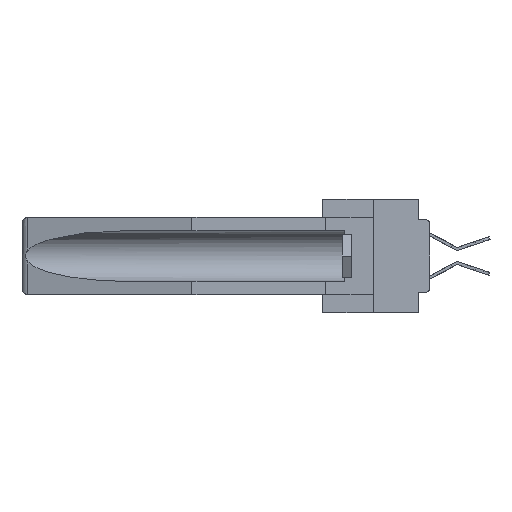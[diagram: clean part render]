
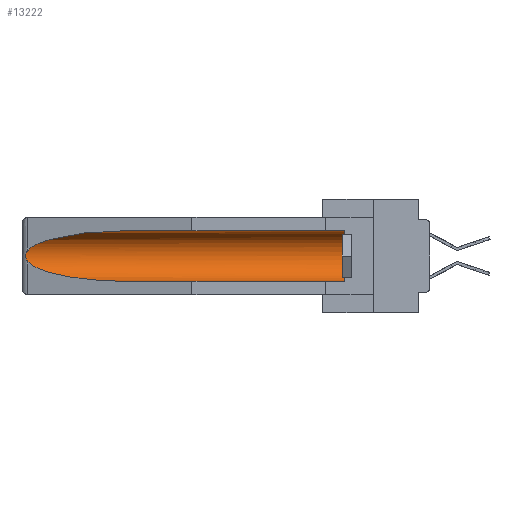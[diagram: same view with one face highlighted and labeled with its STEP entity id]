
A CAD part, left-side view. The second image highlights one B-rep face of the part: STEP entity #13222.
In plain terms, the highlighted cylindrical face has radius 2.857 mm (diameter 5.715 mm), a partial arc.
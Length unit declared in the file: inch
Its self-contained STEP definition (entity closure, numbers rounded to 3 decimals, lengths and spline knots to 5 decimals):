
#59 = CYLINDRICAL_SURFACE ( 'NONE', #3609, 0.1125 ) ;
#587 = CARTESIAN_POINT ( 'NONE',  ( 0.155, 0.126, -0.284 ) ) ;
#2237 = ORIENTED_EDGE ( 'NONE', *, *, #24105, .T. ) ;
#3097 = CARTESIAN_POINT ( 'NONE',  ( 0.26537, 1.52718, -0.19328 ) ) ;
#3282 = VECTOR ( 'NONE', #11240, 39.37008 ) ;
#3609 = AXIS2_PLACEMENT_3D ( 'NONE', #10146, #29214, #24515 ) ;
#4091 = CIRCLE ( 'NONE', #30299, 0.1125 ) ;
#4352 = CARTESIAN_POINT ( 'NONE',  ( 0.155, 1.07973, -0.059 ) ) ;
#4492 = VERTEX_POINT ( 'NONE', #15584 ) ;
#4972 = CARTESIAN_POINT ( 'NONE',  ( 0.26655, 1.53094, -0.18657 ) ) ;
#6360 = EDGE_LOOP ( 'NONE', ( #16870, #11389, #2237, #26771, #13676, #27246 ) ) ;
#6765 = CARTESIAN_POINT ( 'NONE',  ( 0.21114, 1.30732, -0.059 ) ) ;
#6907 = CARTESIAN_POINT ( 'NONE',  ( 0.26597, 1.52961, -0.15275 ) ) ;
#7057 = CARTESIAN_POINT ( 'NONE',  ( 0.2675, 1.53308, -0.17534 ) ) ;
#7318 = CARTESIAN_POINT ( 'NONE',  ( 0.26537, 1.52718, -0.19328 ) ) ;
#7670 = CARTESIAN_POINT ( 'NONE',  ( 0.26597, 1.5296, -0.19026 ) ) ;
#7791 = CARTESIAN_POINT ( 'NONE',  ( 0.155, 1.07973, -0.059 ) ) ;
#8106 = CARTESIAN_POINT ( 'NONE',  ( 0.155, 0.126, -0.1715 ) ) ;
#9405 = CARTESIAN_POINT ( 'NONE',  ( 0.26654, 1.53092, -0.15636 ) ) ;
#10146 = CARTESIAN_POINT ( 'NONE',  ( 0.155, -0.30754, -0.1715 ) ) ;
#10434 = LINE ( 'NONE', #17737, #3282 ) ;
#10909 = VERTEX_POINT ( 'NONE', #587 ) ;
#11240 = DIRECTION ( 'NONE',  ( 0., 1., 0. ) ) ;
#11389 = ORIENTED_EDGE ( 'NONE', *, *, #12657, .T. ) ;
#12652 = VERTEX_POINT ( 'NONE', #13850 ) ;
#12657 = EDGE_CURVE ( 'NONE', #26228, #17143, #29746, .T. ) ;
#13222 = ADVANCED_FACE ( 'NONE', ( #24674 ), #59, .F. ) ;
#13676 = ORIENTED_EDGE ( 'NONE', *, *, #14643, .T. ) ;
#13833 = VECTOR ( 'NONE', #21723, 39.37008 ) ;
#13850 = CARTESIAN_POINT ( 'NONE',  ( 0.155, 0.126, -0.059 ) ) ;
#14643 = EDGE_CURVE ( 'NONE', #10909, #12652, #4091, .T. ) ;
#15046 = CARTESIAN_POINT ( 'NONE',  ( 0.21114, 1.30732, -0.284 ) ) ;
#15584 = CARTESIAN_POINT ( 'NONE',  ( 0.155, 1.07973, -0.284 ) ) ;
#16261 = CARTESIAN_POINT ( 'NONE',  ( 0.26537, 1.52718, -0.14972 ) ) ;
#16856 = EDGE_CURVE ( 'NONE', #21688, #26228, #21368, .T. ) ;
#16870 = ORIENTED_EDGE ( 'NONE', *, *, #16856, .T. ) ;
#16962 = LINE ( 'NONE', #29062, #13833 ) ;
#17143 = VERTEX_POINT ( 'NONE', #3097 ) ;
#17422 = EDGE_CURVE ( 'NONE', #10909, #4492, #16962, .T. ) ;
#17737 = CARTESIAN_POINT ( 'NONE',  ( 0.155, -0.30754, -0.059 ) ) ;
#17745 = DIRECTION ( 'NONE',  ( 0., 0., 1. ) ) ;
#19074 = CARTESIAN_POINT ( 'NONE',  ( 0.2673, 1.5327, -0.16383 ) ) ;
#19543 = CARTESIAN_POINT ( 'NONE',  ( 0.26537, 1.52718, -0.19328 ) ) ;
#21368 =( BOUNDED_CURVE ( )  B_SPLINE_CURVE ( 3, ( #4352, #6765, #28495, #23171 ),
 .UNSPECIFIED., .F., .F. ) 
 B_SPLINE_CURVE_WITH_KNOTS ( ( 4, 4 ),
 ( 4.71239, 6.08839 ),
 .UNSPECIFIED. ) 
 CURVE ( )  GEOMETRIC_REPRESENTATION_ITEM ( )  RATIONAL_B_SPLINE_CURVE ( ( 1., 0.848, 0.848, 1. ) ) 
 REPRESENTATION_ITEM ( '' )  );
#21688 = VERTEX_POINT ( 'NONE', #7791 ) ;
#21723 = DIRECTION ( 'NONE',  ( 0., 1., 0. ) ) ;
#23002 = EDGE_CURVE ( 'NONE', #12652, #21688, #10434, .T. ) ;
#23171 = CARTESIAN_POINT ( 'NONE',  ( 0.26537, 1.52718, -0.14972 ) ) ;
#24105 = EDGE_CURVE ( 'NONE', #17143, #4492, #25926, .T. ) ;
#24515 = DIRECTION ( 'NONE',  ( 0., 0., 1. ) ) ;
#24674 = FACE_OUTER_BOUND ( 'NONE', #6360, .T. ) ;
#25926 =( BOUNDED_CURVE ( )  B_SPLINE_CURVE ( 3, ( #7318, #29527, #15046, #26692 ),
 .UNSPECIFIED., .F., .F. ) 
 B_SPLINE_CURVE_WITH_KNOTS ( ( 4, 4 ),
 ( 0.1948, 1.5708 ),
 .UNSPECIFIED. ) 
 CURVE ( )  GEOMETRIC_REPRESENTATION_ITEM ( )  RATIONAL_B_SPLINE_CURVE ( ( 1., 0.848, 0.848, 1. ) ) 
 REPRESENTATION_ITEM ( '' )  );
#26228 = VERTEX_POINT ( 'NONE', #16261 ) ;
#26692 = CARTESIAN_POINT ( 'NONE',  ( 0.155, 1.07973, -0.284 ) ) ;
#26736 = CARTESIAN_POINT ( 'NONE',  ( 0.2673, 1.53269, -0.17917 ) ) ;
#26771 = ORIENTED_EDGE ( 'NONE', *, *, #17422, .F. ) ;
#27246 = ORIENTED_EDGE ( 'NONE', *, *, #23002, .T. ) ;
#27464 = DIRECTION ( 'NONE',  ( 0., -1., 0. ) ) ;
#28481 = CARTESIAN_POINT ( 'NONE',  ( 0.26537, 1.52718, -0.14972 ) ) ;
#28495 = CARTESIAN_POINT ( 'NONE',  ( 0.25451, 1.48313, -0.09465 ) ) ;
#28631 = CARTESIAN_POINT ( 'NONE',  ( 0.2675, 1.53308, -0.16763 ) ) ;
#29062 = CARTESIAN_POINT ( 'NONE',  ( 0.155, -0.30754, -0.284 ) ) ;
#29214 = DIRECTION ( 'NONE',  ( 0., 1., 0. ) ) ;
#29527 = CARTESIAN_POINT ( 'NONE',  ( 0.25451, 1.48313, -0.24835 ) ) ;
#29746 = B_SPLINE_CURVE_WITH_KNOTS ( 'NONE', 3,
 ( #28481, #6907, #9405, #19074, #28631, #7057, #26736, #4972, #7670, #19543 ),
 .UNSPECIFIED., .F., .F.,
 ( 4, 2, 2, 2, 4 ),
 ( 0., 0.00029, 0.00058, 0.00087, 0.00117 ),
 .UNSPECIFIED. ) ;
#30299 = AXIS2_PLACEMENT_3D ( 'NONE', #8106, #27464, #17745 ) ;
